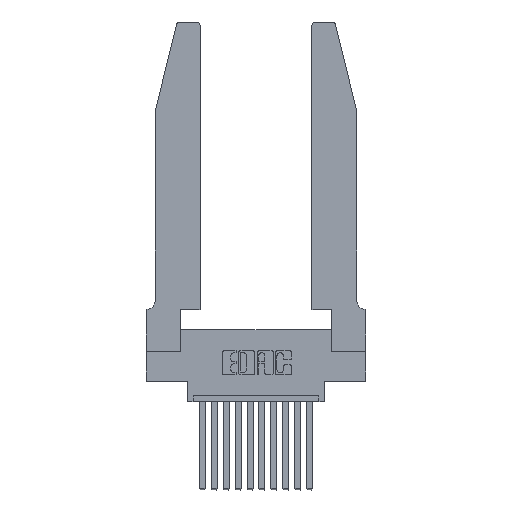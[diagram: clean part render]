
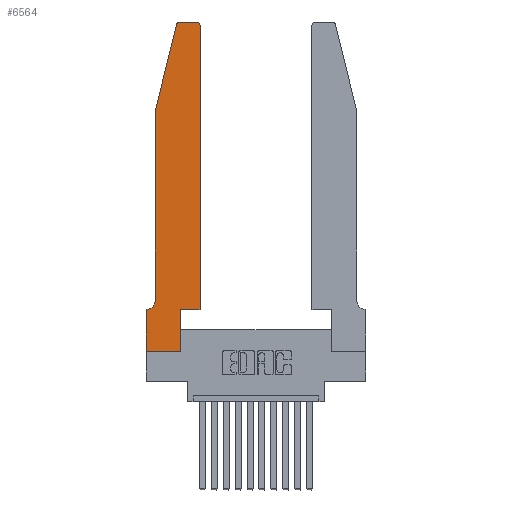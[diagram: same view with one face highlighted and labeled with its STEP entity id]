
A CAD part, top view. The second image highlights one B-rep face of the part: STEP entity #6564.
In plain terms, the highlighted planar face has unit normal (0, 0, 1).
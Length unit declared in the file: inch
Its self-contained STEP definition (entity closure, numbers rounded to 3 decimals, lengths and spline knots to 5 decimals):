
#161 = CARTESIAN_POINT ( 'NONE',  ( 0.2865, 0.35, 0.37 ) ) ;
#408 = CARTESIAN_POINT ( 'NONE',  ( 0., 0., 0.37 ) ) ;
#478 = DIRECTION ( 'NONE',  ( 1., 0., 0. ) ) ;
#563 = EDGE_CURVE ( 'NONE', #12032, #13899, #6960, .T. ) ;
#601 = CARTESIAN_POINT ( 'NONE',  ( 0.284, 2.72, 0.37 ) ) ;
#604 = LINE ( 'NONE', #7321, #13770 ) ;
#2292 = CARTESIAN_POINT ( 'NONE',  ( 0.2605, 2.75, 0.37 ) ) ;
#2400 = EDGE_CURVE ( 'NONE', #13899, #5423, #16427, .T. ) ;
#2591 = DIRECTION ( 'NONE',  ( -1., 0., 0. ) ) ;
#2747 = EDGE_CURVE ( 'NONE', #14844, #9886, #13987, .T. ) ;
#3025 = CARTESIAN_POINT ( 'NONE',  ( 0.4205, 2.72, 0.37 ) ) ;
#3109 = VERTEX_POINT ( 'NONE', #6334 ) ;
#3588 = DIRECTION ( 'NONE',  ( -1., 0., 0. ) ) ;
#3653 = EDGE_CURVE ( 'NONE', #3837, #5417, #5844, .T. ) ;
#3761 = ORIENTED_EDGE ( 'NONE', *, *, #15537, .T. ) ;
#3837 = VERTEX_POINT ( 'NONE', #161 ) ;
#3878 = ORIENTED_EDGE ( 'NONE', *, *, #15921, .T. ) ;
#3889 = FACE_OUTER_BOUND ( 'NONE', #12872, .T. ) ;
#4008 = CARTESIAN_POINT ( 'NONE',  ( 0.4505, 0.35, 0.37 ) ) ;
#4044 = AXIS2_PLACEMENT_3D ( 'NONE', #601, #11931, #8384 ) ;
#4193 = DIRECTION ( 'NONE',  ( 1., 0., 0. ) ) ;
#4200 = VECTOR ( 'NONE', #10495, 39.37008 ) ;
#4703 = DIRECTION ( 'NONE',  ( 1., 0., 0. ) ) ;
#4709 = CIRCLE ( 'NONE', #13388, 0.07 ) ;
#5417 = VERTEX_POINT ( 'NONE', #4008 ) ;
#5423 = VERTEX_POINT ( 'NONE', #12258 ) ;
#5844 = LINE ( 'NONE', #14560, #7848 ) ;
#6002 = LINE ( 'NONE', #8659, #10556 ) ;
#6195 = DIRECTION ( 'NONE',  ( 0., -1., 0. ) ) ;
#6283 = EDGE_CURVE ( 'NONE', #5417, #14844, #14630, .T. ) ;
#6325 = CARTESIAN_POINT ( 'NONE',  ( 0.0755, 0.35, 0.37 ) ) ;
#6334 = CARTESIAN_POINT ( 'NONE',  ( 0.2865, 0., 0.37 ) ) ;
#6406 = CARTESIAN_POINT ( 'NONE',  ( 0.0755, 2., 0.37 ) ) ;
#6564 = ADVANCED_FACE ( 'NONE', ( #3889 ), #14518, .T. ) ;
#6735 = DIRECTION ( 'NONE',  ( -1., 0., 0. ) ) ;
#6799 = ORIENTED_EDGE ( 'NONE', *, *, #3653, .T. ) ;
#6844 = ORIENTED_EDGE ( 'NONE', *, *, #2400, .T. ) ;
#6936 = VERTEX_POINT ( 'NONE', #408 ) ;
#6960 = CIRCLE ( 'NONE', #4044, 0.03 ) ;
#7272 = VECTOR ( 'NONE', #12549, 39.37008 ) ;
#7321 = CARTESIAN_POINT ( 'NONE',  ( 0., 0., 0.37 ) ) ;
#7628 = LINE ( 'NONE', #2292, #12127 ) ;
#7641 = VERTEX_POINT ( 'NONE', #8091 ) ;
#7848 = VECTOR ( 'NONE', #4193, 39.37008 ) ;
#7870 = CARTESIAN_POINT ( 'NONE',  ( 0.284, 2.75, 0.37 ) ) ;
#8058 = CARTESIAN_POINT ( 'NONE',  ( 0.0055, 0.42, 0.37 ) ) ;
#8091 = CARTESIAN_POINT ( 'NONE',  ( 0.0755, 0.42, 0.37 ) ) ;
#8384 = DIRECTION ( 'NONE',  ( 1., 0., 0. ) ) ;
#8556 = CARTESIAN_POINT ( 'NONE',  ( 0.25487, 2.72718, 0.37 ) ) ;
#8659 = CARTESIAN_POINT ( 'NONE',  ( 0.2865, 0.35, 0.37 ) ) ;
#8834 = CARTESIAN_POINT ( 'NONE',  ( 0.4505, 0.35, 0.37 ) ) ;
#9275 = EDGE_CURVE ( 'NONE', #9886, #12032, #7628, .T. ) ;
#9307 = CARTESIAN_POINT ( 'NONE',  ( 0.4505, 2.72, 0.37 ) ) ;
#9351 = CARTESIAN_POINT ( 'NONE',  ( 0., 0., 0.37 ) ) ;
#9594 = LINE ( 'NONE', #9351, #12944 ) ;
#9647 = DIRECTION ( 'NONE',  ( 1., 0., 0. ) ) ;
#9886 = VERTEX_POINT ( 'NONE', #12439 ) ;
#9942 = VERTEX_POINT ( 'NONE', #11123 ) ;
#10065 = VERTEX_POINT ( 'NONE', #10463 ) ;
#10383 = ORIENTED_EDGE ( 'NONE', *, *, #9275, .T. ) ;
#10435 = DIRECTION ( 'NONE',  ( 0., 0., -1. ) ) ;
#10463 = CARTESIAN_POINT ( 'NONE',  ( 0.0055, 0.35, 0.37 ) ) ;
#10495 = DIRECTION ( 'NONE',  ( 0., -1., 0. ) ) ;
#10556 = VECTOR ( 'NONE', #16248, 39.37008 ) ;
#11123 = CARTESIAN_POINT ( 'NONE',  ( 0., 0.35, 0.37 ) ) ;
#11183 = ORIENTED_EDGE ( 'NONE', *, *, #13470, .T. ) ;
#11584 = CARTESIAN_POINT ( 'NONE',  ( 0.0755, 2., 0.37 ) ) ;
#11899 = EDGE_CURVE ( 'NONE', #7641, #10065, #4709, .T. ) ;
#11931 = DIRECTION ( 'NONE',  ( 0., 0., 1. ) ) ;
#12032 = VERTEX_POINT ( 'NONE', #7870 ) ;
#12127 = VECTOR ( 'NONE', #3588, 39.37008 ) ;
#12258 = CARTESIAN_POINT ( 'NONE',  ( 0.0755, 2., 0.37 ) ) ;
#12439 = CARTESIAN_POINT ( 'NONE',  ( 0.4205, 2.75, 0.37 ) ) ;
#12549 = DIRECTION ( 'NONE',  ( -0.239, -0.971, 0. ) ) ;
#12718 = ORIENTED_EDGE ( 'NONE', *, *, #2747, .T. ) ;
#12872 = EDGE_LOOP ( 'NONE', ( #10383, #14733, #6844, #3761, #13851, #11183, #16468, #15546, #3878, #6799, #14048, #12718 ) ) ;
#12944 = VECTOR ( 'NONE', #478, 39.37008 ) ;
#13388 = AXIS2_PLACEMENT_3D ( 'NONE', #8058, #10435, #6735 ) ;
#13470 = EDGE_CURVE ( 'NONE', #10065, #9942, #13633, .T. ) ;
#13633 = LINE ( 'NONE', #6325, #15635 ) ;
#13770 = VECTOR ( 'NONE', #6195, 39.37008 ) ;
#13851 = ORIENTED_EDGE ( 'NONE', *, *, #11899, .T. ) ;
#13899 = VERTEX_POINT ( 'NONE', #8556 ) ;
#13965 = LINE ( 'NONE', #11584, #4200 ) ;
#13987 = CIRCLE ( 'NONE', #15389, 0.03 ) ;
#14048 = ORIENTED_EDGE ( 'NONE', *, *, #6283, .T. ) ;
#14134 = AXIS2_PLACEMENT_3D ( 'NONE', #15973, #14852, #4703 ) ;
#14518 = PLANE ( 'NONE',  #14134 ) ;
#14560 = CARTESIAN_POINT ( 'NONE',  ( 0.4505, 0.35, 0.37 ) ) ;
#14630 = LINE ( 'NONE', #8834, #16412 ) ;
#14733 = ORIENTED_EDGE ( 'NONE', *, *, #563, .T. ) ;
#14844 = VERTEX_POINT ( 'NONE', #9307 ) ;
#14852 = DIRECTION ( 'NONE',  ( 0., 0., 1. ) ) ;
#15082 = EDGE_CURVE ( 'NONE', #6936, #3109, #9594, .T. ) ;
#15125 = DIRECTION ( 'NONE',  ( 0., 1., 0. ) ) ;
#15365 = EDGE_CURVE ( 'NONE', #9942, #6936, #604, .T. ) ;
#15389 = AXIS2_PLACEMENT_3D ( 'NONE', #3025, #15784, #9647 ) ;
#15537 = EDGE_CURVE ( 'NONE', #5423, #7641, #13965, .T. ) ;
#15546 = ORIENTED_EDGE ( 'NONE', *, *, #15082, .T. ) ;
#15635 = VECTOR ( 'NONE', #2591, 39.37008 ) ;
#15784 = DIRECTION ( 'NONE',  ( 0., 0., 1. ) ) ;
#15921 = EDGE_CURVE ( 'NONE', #3109, #3837, #6002, .T. ) ;
#15973 = CARTESIAN_POINT ( 'NONE',  ( 0., 0.35, 0.37 ) ) ;
#16248 = DIRECTION ( 'NONE',  ( 0., 1., 0. ) ) ;
#16412 = VECTOR ( 'NONE', #15125, 39.37008 ) ;
#16427 = LINE ( 'NONE', #6406, #7272 ) ;
#16468 = ORIENTED_EDGE ( 'NONE', *, *, #15365, .T. ) ;
